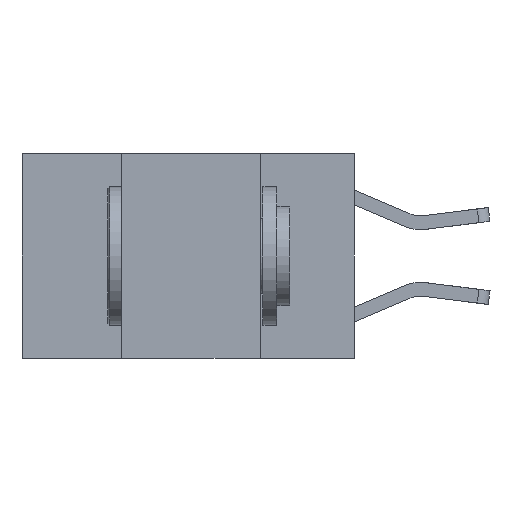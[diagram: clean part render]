
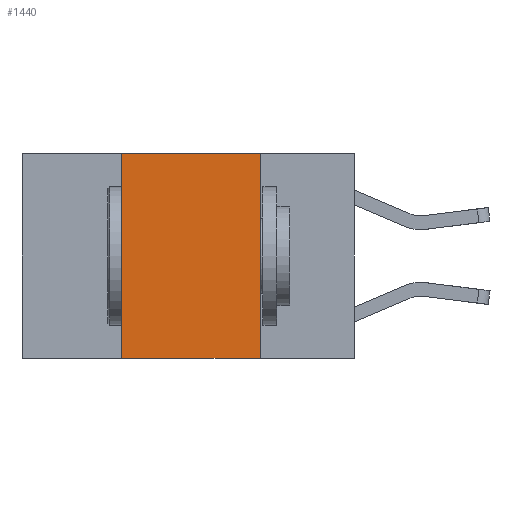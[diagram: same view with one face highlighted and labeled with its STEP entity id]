
A CAD part, left-side view. The second image highlights one B-rep face of the part: STEP entity #1440.
In plain terms, the highlighted planar face has unit normal (-1, 0, 0).
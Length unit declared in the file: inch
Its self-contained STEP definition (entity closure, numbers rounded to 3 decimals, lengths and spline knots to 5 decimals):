
#193 = CARTESIAN_POINT ( 'NONE',  ( 0., 0.42, 0. ) ) ;
#655 = ORIENTED_EDGE ( 'NONE', *, *, #9451, .F. ) ;
#978 = ORIENTED_EDGE ( 'NONE', *, *, #8921, .F. ) ;
#1112 = DIRECTION ( 'NONE',  ( 0., 0., 1. ) ) ;
#1209 = CARTESIAN_POINT ( 'NONE',  ( 0., 0.6, 0. ) ) ;
#1440 = ADVANCED_FACE ( 'NONE', ( #9206 ), #5026, .F. ) ;
#2379 = DIRECTION ( 'NONE',  ( 0., 0., -1. ) ) ;
#2724 = VERTEX_POINT ( 'NONE', #10700 ) ;
#2854 = CARTESIAN_POINT ( 'NONE',  ( 0., 0.42, -0.37 ) ) ;
#3068 = VERTEX_POINT ( 'NONE', #2854 ) ;
#3313 = LINE ( 'NONE', #4268, #9521 ) ;
#3780 = VECTOR ( 'NONE', #3984, 39.37008 ) ;
#3984 = DIRECTION ( 'NONE',  ( 0., -1., 0. ) ) ;
#4140 = ORIENTED_EDGE ( 'NONE', *, *, #7173, .T. ) ;
#4268 = CARTESIAN_POINT ( 'NONE',  ( 0., 0.17, 0. ) ) ;
#4618 = ORIENTED_EDGE ( 'NONE', *, *, #8325, .F. ) ;
#4772 = VERTEX_POINT ( 'NONE', #5197 ) ;
#5026 = PLANE ( 'NONE',  #7984 ) ;
#5133 = DIRECTION ( 'NONE',  ( 0., 0., -1. ) ) ;
#5197 = CARTESIAN_POINT ( 'NONE',  ( 0., 0.42, 0. ) ) ;
#5805 = VECTOR ( 'NONE', #9573, 39.37008 ) ;
#6003 = EDGE_LOOP ( 'NONE', ( #655, #978, #4618, #4140 ) ) ;
#6023 = LINE ( 'NONE', #7352, #3780 ) ;
#7173 = EDGE_CURVE ( 'NONE', #3068, #2724, #6023, .T. ) ;
#7352 = CARTESIAN_POINT ( 'NONE',  ( 0., 0.6, -0.37 ) ) ;
#7984 = AXIS2_PLACEMENT_3D ( 'NONE', #1209, #9948, #2379 ) ;
#8096 = LINE ( 'NONE', #9537, #5805 ) ;
#8218 = VECTOR ( 'NONE', #1112, 39.37008 ) ;
#8325 = EDGE_CURVE ( 'NONE', #3068, #4772, #10684, .T. ) ;
#8921 = EDGE_CURVE ( 'NONE', #4772, #9654, #8096, .T. ) ;
#9206 = FACE_OUTER_BOUND ( 'NONE', #6003, .T. ) ;
#9451 = EDGE_CURVE ( 'NONE', #9654, #2724, #3313, .T. ) ;
#9521 = VECTOR ( 'NONE', #5133, 39.37008 ) ;
#9537 = CARTESIAN_POINT ( 'NONE',  ( 0., 0.6, 0. ) ) ;
#9573 = DIRECTION ( 'NONE',  ( 0., -1., 0. ) ) ;
#9595 = CARTESIAN_POINT ( 'NONE',  ( 0., 0.17, 0. ) ) ;
#9654 = VERTEX_POINT ( 'NONE', #9595 ) ;
#9948 = DIRECTION ( 'NONE',  ( 1., 0., 0. ) ) ;
#10684 = LINE ( 'NONE', #193, #8218 ) ;
#10700 = CARTESIAN_POINT ( 'NONE',  ( 0., 0.17, -0.37 ) ) ;
